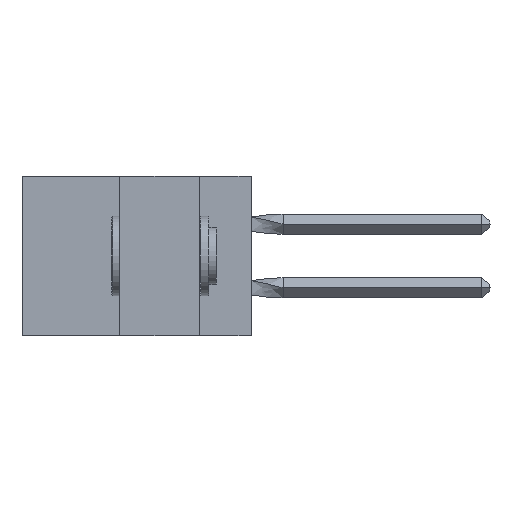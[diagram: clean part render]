
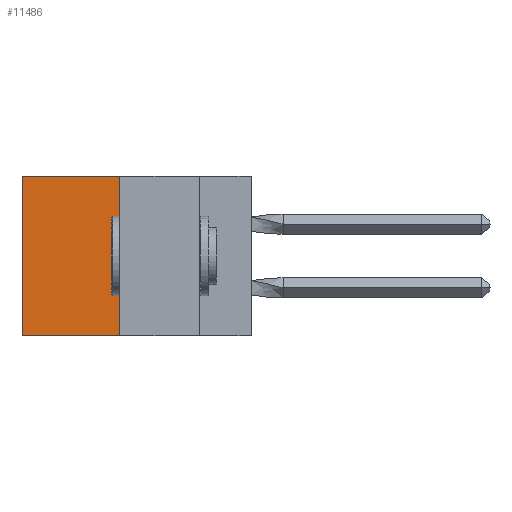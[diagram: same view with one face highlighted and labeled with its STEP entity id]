
A CAD part, left-side view. The second image highlights one B-rep face of the part: STEP entity #11486.
In plain terms, the highlighted planar face has unit normal (-1, 0, 0).
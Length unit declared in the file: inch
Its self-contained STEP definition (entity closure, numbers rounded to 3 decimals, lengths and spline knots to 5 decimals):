
#40 = LINE ( 'NONE', #2622, #7874 ) ;
#234 = CARTESIAN_POINT ( 'NONE',  ( 0.305, 0.413, 0. ) ) ;
#252 = DIRECTION ( 'NONE',  ( 0., 1., 0. ) ) ;
#834 = DIRECTION ( 'NONE',  ( 1., 0., 0. ) ) ;
#890 = CARTESIAN_POINT ( 'NONE',  ( 0.305, 0.413, -0.5 ) ) ;
#1083 = VERTEX_POINT ( 'NONE', #890 ) ;
#2622 = CARTESIAN_POINT ( 'NONE',  ( 0.305, 0.413, -0.5 ) ) ;
#2660 = EDGE_CURVE ( 'NONE', #11153, #14350, #12133, .T. ) ;
#2756 = AXIS2_PLACEMENT_3D ( 'NONE', #11669, #834, #10861 ) ;
#2766 = VECTOR ( 'NONE', #5950, 39.37008 ) ;
#2829 = PLANE ( 'NONE',  #2756 ) ;
#4075 = CARTESIAN_POINT ( 'NONE',  ( 0.305, 0.72, -0.5 ) ) ;
#4126 = DIRECTION ( 'NONE',  ( 0., 0., -1. ) ) ;
#4196 = FACE_OUTER_BOUND ( 'NONE', #7236, .T. ) ;
#4590 = CARTESIAN_POINT ( 'NONE',  ( 0.305, 0.72, 0. ) ) ;
#4860 = VECTOR ( 'NONE', #4126, 39.37008 ) ;
#5501 = EDGE_CURVE ( 'NONE', #11235, #1083, #6432, .T. ) ;
#5950 = DIRECTION ( 'NONE',  ( 0., 0., -1. ) ) ;
#6139 = CARTESIAN_POINT ( 'NONE',  ( 0.305, 0.413, -0.5 ) ) ;
#6432 = LINE ( 'NONE', #6139, #2766 ) ;
#6807 = ORIENTED_EDGE ( 'NONE', *, *, #11711, .F. ) ;
#7236 = EDGE_LOOP ( 'NONE', ( #10909, #6807, #7790, #8954 ) ) ;
#7382 = VECTOR ( 'NONE', #13400, 39.37008 ) ;
#7790 = ORIENTED_EDGE ( 'NONE', *, *, #5501, .F. ) ;
#7874 = VECTOR ( 'NONE', #252, 39.37008 ) ;
#8954 = ORIENTED_EDGE ( 'NONE', *, *, #10296, .T. ) ;
#10296 = EDGE_CURVE ( 'NONE', #11235, #11153, #13918, .T. ) ;
#10390 = CARTESIAN_POINT ( 'NONE',  ( 0.305, 0.413, 0. ) ) ;
#10861 = DIRECTION ( 'NONE',  ( 0., 0., -1. ) ) ;
#10909 = ORIENTED_EDGE ( 'NONE', *, *, #2660, .T. ) ;
#11153 = VERTEX_POINT ( 'NONE', #4590 ) ;
#11235 = VERTEX_POINT ( 'NONE', #10390 ) ;
#11486 = ADVANCED_FACE ( 'NONE', ( #4196 ), #2829, .F. ) ;
#11669 = CARTESIAN_POINT ( 'NONE',  ( 0.305, 0.413, -0.5 ) ) ;
#11711 = EDGE_CURVE ( 'NONE', #1083, #14350, #40, .T. ) ;
#12133 = LINE ( 'NONE', #4075, #4860 ) ;
#12995 = CARTESIAN_POINT ( 'NONE',  ( 0.305, 0.72, -0.5 ) ) ;
#13400 = DIRECTION ( 'NONE',  ( 0., 1., 0. ) ) ;
#13918 = LINE ( 'NONE', #234, #7382 ) ;
#14350 = VERTEX_POINT ( 'NONE', #12995 ) ;
